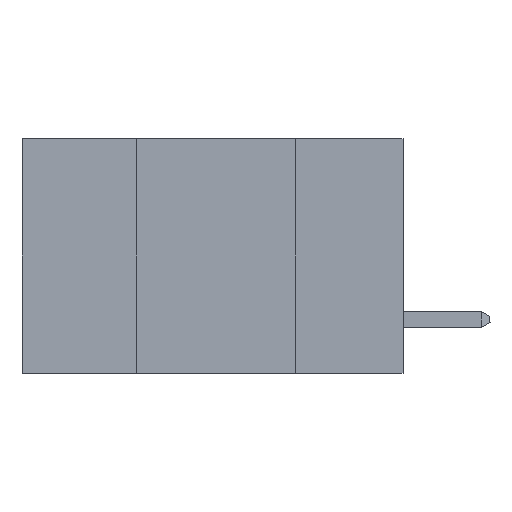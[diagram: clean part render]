
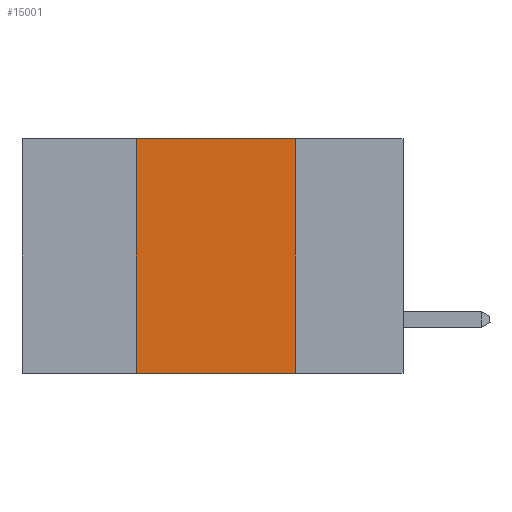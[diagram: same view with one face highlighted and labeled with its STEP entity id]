
A CAD part, left-side view. The second image highlights one B-rep face of the part: STEP entity #15001.
In plain terms, the highlighted planar face has unit normal (-1, 0, 0).
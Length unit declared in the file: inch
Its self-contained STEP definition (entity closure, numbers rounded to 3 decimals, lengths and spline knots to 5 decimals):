
#964 = VECTOR ( 'NONE', #37257, 39.37008 ) ;
#1286 = VERTEX_POINT ( 'NONE', #10966 ) ;
#1324 = DIRECTION ( 'NONE',  ( 0., 0., -1. ) ) ;
#1404 = CARTESIAN_POINT ( 'NONE',  ( 0., 0.6, 0. ) ) ;
#3324 = EDGE_CURVE ( 'NONE', #19286, #29351, #43221, .T. ) ;
#4518 = VERTEX_POINT ( 'NONE', #14816 ) ;
#5960 = EDGE_CURVE ( 'NONE', #29351, #4518, #15739, .T. ) ;
#7065 = CARTESIAN_POINT ( 'NONE',  ( 0., 0.17, 0. ) ) ;
#7146 = CARTESIAN_POINT ( 'NONE',  ( 0., 0.6, -0.37 ) ) ;
#8287 = CARTESIAN_POINT ( 'NONE',  ( 0., 0.42, 0. ) ) ;
#8825 = ORIENTED_EDGE ( 'NONE', *, *, #16207, .T. ) ;
#10750 = EDGE_CURVE ( 'NONE', #1286, #19286, #30517, .T. ) ;
#10966 = CARTESIAN_POINT ( 'NONE',  ( 0., 0.42, -0.37 ) ) ;
#14173 = CARTESIAN_POINT ( 'NONE',  ( 0., 0.6, 0. ) ) ;
#14310 = DIRECTION ( 'NONE',  ( 1., 0., 0. ) ) ;
#14816 = CARTESIAN_POINT ( 'NONE',  ( 0., 0.17, -0.37 ) ) ;
#15001 = ADVANCED_FACE ( 'NONE', ( #42619 ), #41233, .F. ) ;
#15739 = LINE ( 'NONE', #7065, #964 ) ;
#16207 = EDGE_CURVE ( 'NONE', #1286, #4518, #16308, .T. ) ;
#16308 = LINE ( 'NONE', #7146, #34667 ) ;
#17957 = ORIENTED_EDGE ( 'NONE', *, *, #10750, .F. ) ;
#19286 = VERTEX_POINT ( 'NONE', #8287 ) ;
#20194 = VECTOR ( 'NONE', #21707, 39.37008 ) ;
#21707 = DIRECTION ( 'NONE',  ( 0., -1., 0. ) ) ;
#24864 = ORIENTED_EDGE ( 'NONE', *, *, #3324, .F. ) ;
#27076 = AXIS2_PLACEMENT_3D ( 'NONE', #14173, #14310, #1324 ) ;
#28166 = EDGE_LOOP ( 'NONE', ( #42210, #24864, #17957, #8825 ) ) ;
#29351 = VERTEX_POINT ( 'NONE', #31091 ) ;
#30517 = LINE ( 'NONE', #39132, #40449 ) ;
#30625 = DIRECTION ( 'NONE',  ( 0., -1., 0. ) ) ;
#31091 = CARTESIAN_POINT ( 'NONE',  ( 0., 0.17, 0. ) ) ;
#34667 = VECTOR ( 'NONE', #30625, 39.37008 ) ;
#35734 = DIRECTION ( 'NONE',  ( 0., 0., 1. ) ) ;
#37257 = DIRECTION ( 'NONE',  ( 0., 0., -1. ) ) ;
#39132 = CARTESIAN_POINT ( 'NONE',  ( 0., 0.42, 0. ) ) ;
#40449 = VECTOR ( 'NONE', #35734, 39.37008 ) ;
#41233 = PLANE ( 'NONE',  #27076 ) ;
#42210 = ORIENTED_EDGE ( 'NONE', *, *, #5960, .F. ) ;
#42619 = FACE_OUTER_BOUND ( 'NONE', #28166, .T. ) ;
#43221 = LINE ( 'NONE', #1404, #20194 ) ;
